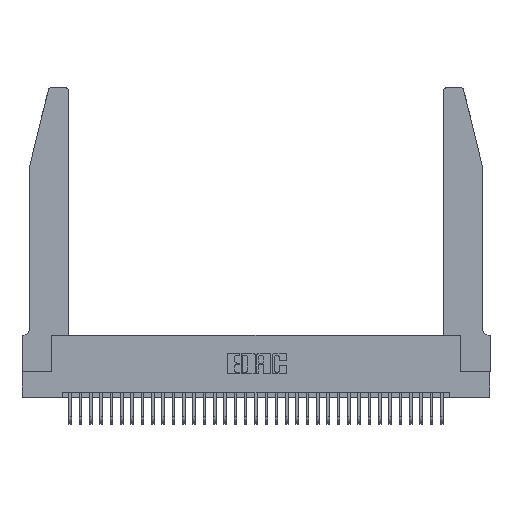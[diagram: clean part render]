
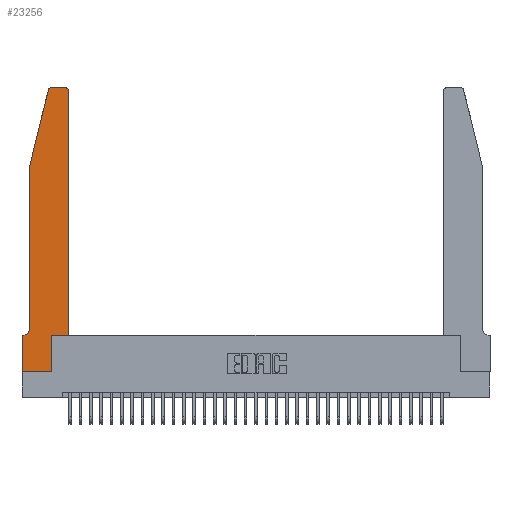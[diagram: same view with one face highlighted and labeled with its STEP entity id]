
A CAD part, top view. The second image highlights one B-rep face of the part: STEP entity #23256.
In plain terms, the highlighted planar face has unit normal (0, 0, 1).
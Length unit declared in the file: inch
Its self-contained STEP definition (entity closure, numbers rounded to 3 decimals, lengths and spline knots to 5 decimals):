
#261 = CARTESIAN_POINT ( 'NONE',  ( 0., 0., 0.37 ) ) ;
#541 = ORIENTED_EDGE ( 'NONE', *, *, #13202, .T. ) ;
#647 = VERTEX_POINT ( 'NONE', #22884 ) ;
#1372 = AXIS2_PLACEMENT_3D ( 'NONE', #4399, #24080, #7276 ) ;
#2107 = ORIENTED_EDGE ( 'NONE', *, *, #9314, .T. ) ;
#2123 = DIRECTION ( 'NONE',  ( -1., 0., 0. ) ) ;
#2190 = EDGE_CURVE ( 'NONE', #24531, #8951, #14387, .T. ) ;
#2470 = CARTESIAN_POINT ( 'NONE',  ( 0.4205, 2.75, 0.37 ) ) ;
#2535 = ORIENTED_EDGE ( 'NONE', *, *, #33100, .T. ) ;
#2559 = LINE ( 'NONE', #7673, #16667 ) ;
#3527 = LINE ( 'NONE', #35711, #10193 ) ;
#3787 = EDGE_CURVE ( 'NONE', #30908, #5812, #3527, .T. ) ;
#4399 = CARTESIAN_POINT ( 'NONE',  ( 0., 0.35, 0.37 ) ) ;
#4548 = DIRECTION ( 'NONE',  ( -1., 0., 0. ) ) ;
#4569 = ORIENTED_EDGE ( 'NONE', *, *, #32820, .T. ) ;
#4721 = VERTEX_POINT ( 'NONE', #14129 ) ;
#5207 = CARTESIAN_POINT ( 'NONE',  ( 0.4505, 2.72, 0.37 ) ) ;
#5812 = VERTEX_POINT ( 'NONE', #12958 ) ;
#5921 = EDGE_CURVE ( 'NONE', #647, #28715, #2559, .T. ) ;
#6292 = CIRCLE ( 'NONE', #7999, 0.07 ) ;
#7276 = DIRECTION ( 'NONE',  ( 1., 0., 0. ) ) ;
#7470 = VECTOR ( 'NONE', #26812, 39.37008 ) ;
#7673 = CARTESIAN_POINT ( 'NONE',  ( 0.0755, 0.35, 0.37 ) ) ;
#7719 = ORIENTED_EDGE ( 'NONE', *, *, #31662, .T. ) ;
#7893 = EDGE_LOOP ( 'NONE', ( #2107, #541, #30793, #10526, #2535, #29730, #4569, #22746, #33669, #7719, #33371, #8055 ) ) ;
#7999 = AXIS2_PLACEMENT_3D ( 'NONE', #35517, #19008, #2123 ) ;
#8055 = ORIENTED_EDGE ( 'NONE', *, *, #2190, .T. ) ;
#8397 = FACE_OUTER_BOUND ( 'NONE', #7893, .T. ) ;
#8534 = CARTESIAN_POINT ( 'NONE',  ( 0.284, 2.72, 0.37 ) ) ;
#8951 = VERTEX_POINT ( 'NONE', #2470 ) ;
#9314 = EDGE_CURVE ( 'NONE', #8951, #29991, #21250, .T. ) ;
#10193 = VECTOR ( 'NONE', #19230, 39.37008 ) ;
#10203 = LINE ( 'NONE', #23365, #16782 ) ;
#10314 = LINE ( 'NONE', #261, #30810 ) ;
#10526 = ORIENTED_EDGE ( 'NONE', *, *, #34198, .T. ) ;
#10722 = CARTESIAN_POINT ( 'NONE',  ( 0.284, 2.75, 0.37 ) ) ;
#11344 = CARTESIAN_POINT ( 'NONE',  ( 0.4505, 0.35, 0.37 ) ) ;
#11386 = DIRECTION ( 'NONE',  ( 1., 0., 0. ) ) ;
#12081 = CIRCLE ( 'NONE', #23879, 0.03 ) ;
#12958 = CARTESIAN_POINT ( 'NONE',  ( 0.0755, 2., 0.37 ) ) ;
#13202 = EDGE_CURVE ( 'NONE', #29991, #30908, #12081, .T. ) ;
#14129 = CARTESIAN_POINT ( 'NONE',  ( 0.2865, 0., 0.37 ) ) ;
#14152 = CARTESIAN_POINT ( 'NONE',  ( 0.4205, 2.72, 0.37 ) ) ;
#14387 = CIRCLE ( 'NONE', #22496, 0.03 ) ;
#15573 = CARTESIAN_POINT ( 'NONE',  ( 0., 0., 0.37 ) ) ;
#15871 = VECTOR ( 'NONE', #16971, 39.37008 ) ;
#16149 = DIRECTION ( 'NONE',  ( -1., 0., 0. ) ) ;
#16667 = VECTOR ( 'NONE', #16149, 39.37008 ) ;
#16782 = VECTOR ( 'NONE', #28923, 39.37008 ) ;
#16971 = DIRECTION ( 'NONE',  ( 0., 1., 0. ) ) ;
#16998 = DIRECTION ( 'NONE',  ( 1., 0., 0. ) ) ;
#17270 = CARTESIAN_POINT ( 'NONE',  ( 0.2865, 0.35, 0.37 ) ) ;
#17427 = LINE ( 'NONE', #20445, #23117 ) ;
#18645 = EDGE_CURVE ( 'NONE', #4721, #20806, #35789, .T. ) ;
#19008 = DIRECTION ( 'NONE',  ( 0., 0., -1. ) ) ;
#19230 = DIRECTION ( 'NONE',  ( -0.239, -0.971, 0. ) ) ;
#20376 = VECTOR ( 'NONE', #4548, 39.37008 ) ;
#20445 = CARTESIAN_POINT ( 'NONE',  ( 0.4505, 0.35, 0.37 ) ) ;
#20806 = VERTEX_POINT ( 'NONE', #17270 ) ;
#21250 = LINE ( 'NONE', #24227, #20376 ) ;
#22496 = AXIS2_PLACEMENT_3D ( 'NONE', #14152, #33615, #16998 ) ;
#22746 = ORIENTED_EDGE ( 'NONE', *, *, #28706, .T. ) ;
#22816 = CARTESIAN_POINT ( 'NONE',  ( 0.2865, 0.35, 0.37 ) ) ;
#22823 = DIRECTION ( 'NONE',  ( 0., -1., 0. ) ) ;
#22884 = CARTESIAN_POINT ( 'NONE',  ( 0.0055, 0.35, 0.37 ) ) ;
#23117 = VECTOR ( 'NONE', #23267, 39.37008 ) ;
#23256 = ADVANCED_FACE ( 'NONE', ( #8397 ), #35010, .T. ) ;
#23267 = DIRECTION ( 'NONE',  ( 1., 0., 0. ) ) ;
#23272 = CARTESIAN_POINT ( 'NONE',  ( 0.25487, 2.72718, 0.37 ) ) ;
#23365 = CARTESIAN_POINT ( 'NONE',  ( 0.0755, 2., 0.37 ) ) ;
#23879 = AXIS2_PLACEMENT_3D ( 'NONE', #8534, #28106, #11386 ) ;
#24080 = DIRECTION ( 'NONE',  ( 0., 0., 1. ) ) ;
#24227 = CARTESIAN_POINT ( 'NONE',  ( 0.2605, 2.75, 0.37 ) ) ;
#24531 = VERTEX_POINT ( 'NONE', #5207 ) ;
#25164 = CARTESIAN_POINT ( 'NONE',  ( 0., 0., 0.37 ) ) ;
#25592 = DIRECTION ( 'NONE',  ( 0., 1., 0. ) ) ;
#26812 = DIRECTION ( 'NONE',  ( 1., 0., 0. ) ) ;
#27774 = VERTEX_POINT ( 'NONE', #11344 ) ;
#28078 = VERTEX_POINT ( 'NONE', #34742 ) ;
#28106 = DIRECTION ( 'NONE',  ( 0., 0., 1. ) ) ;
#28542 = VECTOR ( 'NONE', #25592, 39.37008 ) ;
#28706 = EDGE_CURVE ( 'NONE', #29596, #4721, #30633, .T. ) ;
#28715 = VERTEX_POINT ( 'NONE', #32362 ) ;
#28923 = DIRECTION ( 'NONE',  ( 0., -1., 0. ) ) ;
#29596 = VERTEX_POINT ( 'NONE', #25164 ) ;
#29730 = ORIENTED_EDGE ( 'NONE', *, *, #5921, .T. ) ;
#29991 = VERTEX_POINT ( 'NONE', #10722 ) ;
#30633 = LINE ( 'NONE', #15573, #7470 ) ;
#30679 = LINE ( 'NONE', #30819, #15871 ) ;
#30793 = ORIENTED_EDGE ( 'NONE', *, *, #3787, .T. ) ;
#30810 = VECTOR ( 'NONE', #22823, 39.37008 ) ;
#30819 = CARTESIAN_POINT ( 'NONE',  ( 0.4505, 0.35, 0.37 ) ) ;
#30908 = VERTEX_POINT ( 'NONE', #23272 ) ;
#31662 = EDGE_CURVE ( 'NONE', #20806, #27774, #17427, .T. ) ;
#32362 = CARTESIAN_POINT ( 'NONE',  ( 0., 0.35, 0.37 ) ) ;
#32820 = EDGE_CURVE ( 'NONE', #28715, #29596, #10314, .T. ) ;
#33100 = EDGE_CURVE ( 'NONE', #28078, #647, #6292, .T. ) ;
#33371 = ORIENTED_EDGE ( 'NONE', *, *, #34673, .T. ) ;
#33615 = DIRECTION ( 'NONE',  ( 0., 0., 1. ) ) ;
#33669 = ORIENTED_EDGE ( 'NONE', *, *, #18645, .T. ) ;
#34198 = EDGE_CURVE ( 'NONE', #5812, #28078, #10203, .T. ) ;
#34673 = EDGE_CURVE ( 'NONE', #27774, #24531, #30679, .T. ) ;
#34742 = CARTESIAN_POINT ( 'NONE',  ( 0.0755, 0.42, 0.37 ) ) ;
#35010 = PLANE ( 'NONE',  #1372 ) ;
#35517 = CARTESIAN_POINT ( 'NONE',  ( 0.0055, 0.42, 0.37 ) ) ;
#35711 = CARTESIAN_POINT ( 'NONE',  ( 0.0755, 2., 0.37 ) ) ;
#35789 = LINE ( 'NONE', #22816, #28542 ) ;
